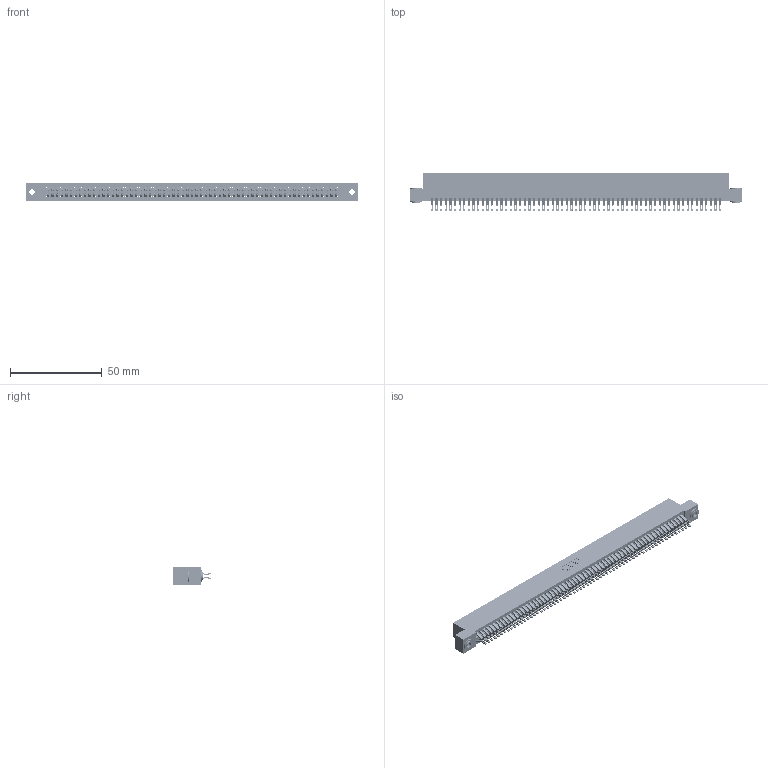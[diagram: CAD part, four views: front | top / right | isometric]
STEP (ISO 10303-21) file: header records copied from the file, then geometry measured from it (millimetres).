
FILE_DESCRIPTION (( 'STEP AP203' ), '1' );
FILE_NAME ('345-126-555-203.STEP', '2019-11-07T04:54:20', ( '' ), ( '' ), 'SwSTEP 2.0', 'SolidWorks 2016', '' );
FILE_SCHEMA (( 'CONFIG_CONTROL_DESIGN' ));
Length unit declared in the file: inch
Products named in the file (4): 345-292-001_555 Tail; 345-126-555-203; 345 Part_Flush Mounting Lugs - 0.156 Dia-TH; 345-250-002_345-250-002-102
Assembly tree (129 placements, depth 2):
  345-126-555-203
    345 Part_Flush Mounting Lugs - 0.156 Dia-TH
    345-292-001_555 Tail  x126
    345-250-002_345-250-002-102  x2
Bounding box: 181.23 x 21.13 x 9.4 mm (x, y, z)
Volume: 18184.6 mm3; surface area: 28762.6 mm2
Topology: 129 solids, 129 shells, 7220 faces, 22719 edges, 15142 vertices
Faces by surface type: plane 3996, cylinder 3216, cone 8
Entity records: 47580 total; most frequent: CARTESIAN_POINT 7965, ORIENTED_EDGE 7862, DIRECTION 6997, EDGE_CURVE 3931, VECTOR 3503, LINE 3503, VERTEX_POINT 2618, AXIS2_PLACEMENT_3D 1747
